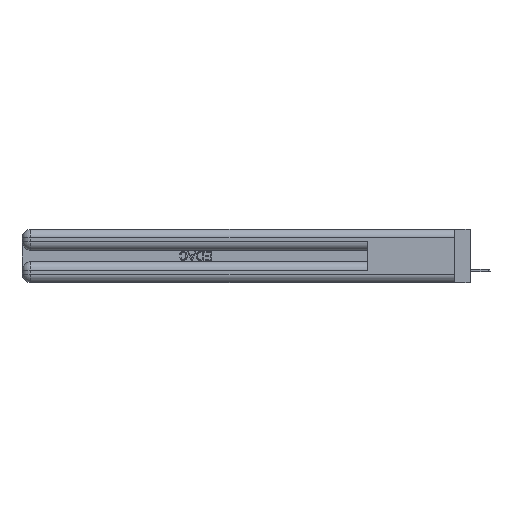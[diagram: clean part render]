
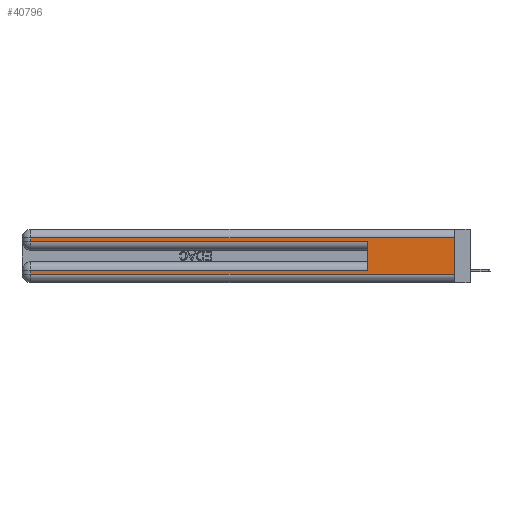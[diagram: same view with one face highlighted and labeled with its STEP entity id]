
A CAD part, left-side view. The second image highlights one B-rep face of the part: STEP entity #40796.
In plain terms, the highlighted planar face has unit normal (-1, 0, 0).
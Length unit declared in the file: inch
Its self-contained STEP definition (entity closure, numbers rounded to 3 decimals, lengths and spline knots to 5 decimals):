
#117 = DIRECTION ( 'NONE',  ( 0., -1., 0. ) ) ;
#250 = LINE ( 'NONE', #26489, #18058 ) ;
#430 = VECTOR ( 'NONE', #31345, 39.37008 ) ;
#768 = CARTESIAN_POINT ( 'NONE',  ( 0., 0.6, 0.085 ) ) ;
#948 = LINE ( 'NONE', #20499, #35658 ) ;
#1037 = EDGE_CURVE ( 'NONE', #7762, #42112, #20392, .T. ) ;
#2053 = CARTESIAN_POINT ( 'NONE',  ( 0., 2.94, 0.31 ) ) ;
#3792 = LINE ( 'NONE', #30036, #4952 ) ;
#4055 = CARTESIAN_POINT ( 'NONE',  ( 0., 0., 0.31 ) ) ;
#4952 = VECTOR ( 'NONE', #117, 39.37008 ) ;
#5027 = ORIENTED_EDGE ( 'NONE', *, *, #34276, .T. ) ;
#5118 = EDGE_CURVE ( 'NONE', #7316, #6600, #19914, .T. ) ;
#5689 = CARTESIAN_POINT ( 'NONE',  ( 0., 2.94, 0.06 ) ) ;
#5734 = DIRECTION ( 'NONE',  ( 0., 0., -1. ) ) ;
#6600 = VERTEX_POINT ( 'NONE', #2053 ) ;
#7316 = VERTEX_POINT ( 'NONE', #4055 ) ;
#7762 = VERTEX_POINT ( 'NONE', #768 ) ;
#9644 = CARTESIAN_POINT ( 'NONE',  ( 0., 0., 0.085 ) ) ;
#9714 = VECTOR ( 'NONE', #13716, 39.37008 ) ;
#10760 = ORIENTED_EDGE ( 'NONE', *, *, #1037, .T. ) ;
#11389 = CARTESIAN_POINT ( 'NONE',  ( 0., 2.94, 0.085 ) ) ;
#13636 = AXIS2_PLACEMENT_3D ( 'NONE', #17981, #24691, #5734 ) ;
#13716 = DIRECTION ( 'NONE',  ( 0., 1., 0. ) ) ;
#14291 = LINE ( 'NONE', #14493, #21178 ) ;
#14493 = CARTESIAN_POINT ( 'NONE',  ( 0., 2.94, 0.37 ) ) ;
#14947 = CARTESIAN_POINT ( 'NONE',  ( 0., 0.6, 0.145 ) ) ;
#15562 = ORIENTED_EDGE ( 'NONE', *, *, #5118, .T. ) ;
#15954 = ORIENTED_EDGE ( 'NONE', *, *, #29348, .F. ) ;
#17774 = VERTEX_POINT ( 'NONE', #5689 ) ;
#17981 = CARTESIAN_POINT ( 'NONE',  ( 0., 0., 0.37 ) ) ;
#18058 = VECTOR ( 'NONE', #39653, 39.37008 ) ;
#18518 = VERTEX_POINT ( 'NONE', #36405 ) ;
#19914 = LINE ( 'NONE', #23797, #24328 ) ;
#20392 = LINE ( 'NONE', #9644, #9714 ) ;
#20499 = CARTESIAN_POINT ( 'NONE',  ( 0., 2.94, 0.37 ) ) ;
#20662 = EDGE_LOOP ( 'NONE', ( #35486, #15562, #5027, #25884, #15954, #10760, #32419, #33434 ) ) ;
#21178 = VECTOR ( 'NONE', #24436, 39.37008 ) ;
#23697 = LINE ( 'NONE', #40500, #30575 ) ;
#23797 = CARTESIAN_POINT ( 'NONE',  ( 0., 0., 0.31 ) ) ;
#24328 = VECTOR ( 'NONE', #39556, 39.37008 ) ;
#24436 = DIRECTION ( 'NONE',  ( 0., 0., -1. ) ) ;
#24516 = EDGE_CURVE ( 'NONE', #7316, #28275, #250, .T. ) ;
#24691 = DIRECTION ( 'NONE',  ( 1., 0., 0. ) ) ;
#25884 = ORIENTED_EDGE ( 'NONE', *, *, #25949, .T. ) ;
#25949 = EDGE_CURVE ( 'NONE', #18518, #33012, #23697, .T. ) ;
#25955 = CARTESIAN_POINT ( 'NONE',  ( 0., 0.6, 0.285 ) ) ;
#26489 = CARTESIAN_POINT ( 'NONE',  ( 0., 0., 0.37 ) ) ;
#26762 = DIRECTION ( 'NONE',  ( 0., 0., -1. ) ) ;
#28275 = VERTEX_POINT ( 'NONE', #33629 ) ;
#29348 = EDGE_CURVE ( 'NONE', #7762, #33012, #31549, .T. ) ;
#30036 = CARTESIAN_POINT ( 'NONE',  ( 0., 0., 0.06 ) ) ;
#30575 = VECTOR ( 'NONE', #40716, 39.37008 ) ;
#31345 = DIRECTION ( 'NONE',  ( 0., 0., 1. ) ) ;
#31549 = LINE ( 'NONE', #14947, #430 ) ;
#32419 = ORIENTED_EDGE ( 'NONE', *, *, #34696, .T. ) ;
#33012 = VERTEX_POINT ( 'NONE', #25955 ) ;
#33434 = ORIENTED_EDGE ( 'NONE', *, *, #37908, .T. ) ;
#33629 = CARTESIAN_POINT ( 'NONE',  ( 0., 0., 0.06 ) ) ;
#34276 = EDGE_CURVE ( 'NONE', #6600, #18518, #14291, .T. ) ;
#34696 = EDGE_CURVE ( 'NONE', #42112, #17774, #948, .T. ) ;
#35218 = FACE_OUTER_BOUND ( 'NONE', #20662, .T. ) ;
#35486 = ORIENTED_EDGE ( 'NONE', *, *, #24516, .F. ) ;
#35658 = VECTOR ( 'NONE', #26762, 39.37008 ) ;
#36405 = CARTESIAN_POINT ( 'NONE',  ( 0., 2.94, 0.285 ) ) ;
#37609 = PLANE ( 'NONE',  #13636 ) ;
#37908 = EDGE_CURVE ( 'NONE', #17774, #28275, #3792, .T. ) ;
#39556 = DIRECTION ( 'NONE',  ( 0., 1., 0. ) ) ;
#39653 = DIRECTION ( 'NONE',  ( 0., 0., -1. ) ) ;
#40500 = CARTESIAN_POINT ( 'NONE',  ( 0., 0., 0.285 ) ) ;
#40716 = DIRECTION ( 'NONE',  ( 0., -1., 0. ) ) ;
#40796 = ADVANCED_FACE ( 'NONE', ( #35218 ), #37609, .F. ) ;
#42112 = VERTEX_POINT ( 'NONE', #11389 ) ;
